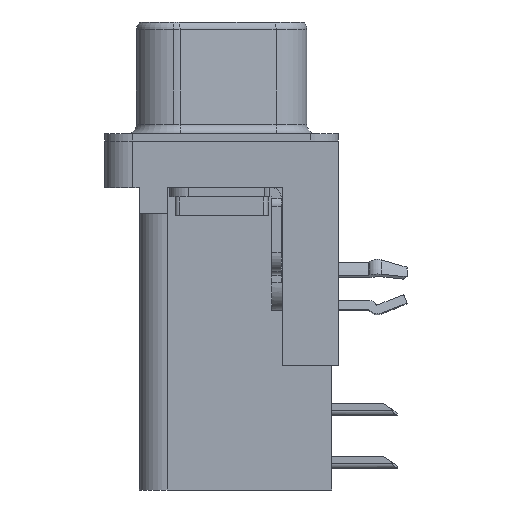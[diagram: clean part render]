
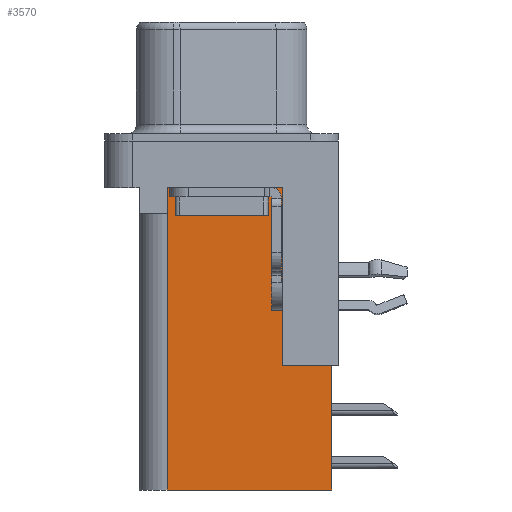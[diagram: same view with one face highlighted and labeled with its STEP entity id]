
A CAD part, left-side view. The second image highlights one B-rep face of the part: STEP entity #3570.
In plain terms, the highlighted planar face has unit normal (-1, 0, 0).
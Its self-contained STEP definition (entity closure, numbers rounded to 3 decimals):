
#552 = VERTEX_POINT ( 'NONE', #10176 ) ;
#607 = VECTOR ( 'NONE', #13355, 1000. ) ;
#747 = LINE ( 'NONE', #12191, #607 ) ;
#1044 = ORIENTED_EDGE ( 'NONE', *, *, #6410, .T. ) ;
#1536 = VECTOR ( 'NONE', #13078, 1000. ) ;
#1740 = LINE ( 'NONE', #16534, #1536 ) ;
#2386 = AXIS2_PLACEMENT_3D ( 'NONE', #10855, #15458, #12419 ) ;
#3159 = ORIENTED_EDGE ( 'NONE', *, *, #15242, .T. ) ;
#3570 = ADVANCED_FACE ( 'NONE', ( #6149 ), #14655, .F. ) ;
#4146 = CARTESIAN_POINT ( 'NONE',  ( 3.765, 2.925, -3.9 ) ) ;
#4366 = DIRECTION ( 'NONE',  ( 0., 0., 1. ) ) ;
#4608 = EDGE_CURVE ( 'NONE', #5738, #17098, #1740, .T. ) ;
#4900 = EDGE_CURVE ( 'NONE', #14322, #7651, #747, .T. ) ;
#4999 = VECTOR ( 'NONE', #13745, 1000. ) ;
#5017 = LINE ( 'NONE', #19969, #4999 ) ;
#5036 = VECTOR ( 'NONE', #10395, 1000. ) ;
#5080 = LINE ( 'NONE', #10647, #5036 ) ;
#5152 = ORIENTED_EDGE ( 'NONE', *, *, #4608, .F. ) ;
#5738 = VERTEX_POINT ( 'NONE', #12251 ) ;
#6149 = FACE_OUTER_BOUND ( 'NONE', #19801, .T. ) ;
#6338 = EDGE_CURVE ( 'NONE', #12247, #6940, #16117, .T. ) ;
#6410 = EDGE_CURVE ( 'NONE', #12247, #552, #15913, .T. ) ;
#6684 = EDGE_CURVE ( 'NONE', #552, #9245, #14926, .T. ) ;
#6762 = ORIENTED_EDGE ( 'NONE', *, *, #11816, .F. ) ;
#6940 = VERTEX_POINT ( 'NONE', #13291 ) ;
#7565 = CARTESIAN_POINT ( 'NONE',  ( 3.765, -3.295, -18.76 ) ) ;
#7651 = VERTEX_POINT ( 'NONE', #13433 ) ;
#7776 = CARTESIAN_POINT ( 'NONE',  ( 3.765, -5.925, -12.05 ) ) ;
#9237 = EDGE_CURVE ( 'NONE', #7651, #17098, #5080, .T. ) ;
#9245 = VERTEX_POINT ( 'NONE', #10326 ) ;
#10036 = CARTESIAN_POINT ( 'NONE',  ( 3.765, -3.295, -18.76 ) ) ;
#10176 = CARTESIAN_POINT ( 'NONE',  ( 3.765, -3.295, -12.05 ) ) ;
#10326 = CARTESIAN_POINT ( 'NONE',  ( 3.765, -3.295, -2.5 ) ) ;
#10370 = ORIENTED_EDGE ( 'NONE', *, *, #6338, .F. ) ;
#10395 = DIRECTION ( 'NONE',  ( 0., 1., 0. ) ) ;
#10647 = CARTESIAN_POINT ( 'NONE',  ( 3.765, 0., -3.9 ) ) ;
#10855 = CARTESIAN_POINT ( 'NONE',  ( 3.765, -3.295, -18.76 ) ) ;
#11762 = DIRECTION ( 'NONE',  ( 0., 1., 0. ) ) ;
#11816 = EDGE_CURVE ( 'NONE', #6940, #5738, #16955, .T. ) ;
#12191 = CARTESIAN_POINT ( 'NONE',  ( 3.765, 2.895, -3.9 ) ) ;
#12247 = VERTEX_POINT ( 'NONE', #7776 ) ;
#12251 = CARTESIAN_POINT ( 'NONE',  ( 3.765, 2.925, -18.76 ) ) ;
#12419 = DIRECTION ( 'NONE',  ( 0., 1., 0. ) ) ;
#13022 = CARTESIAN_POINT ( 'NONE',  ( 3.765, -6.295, -12.05 ) ) ;
#13078 = DIRECTION ( 'NONE',  ( 0., 0., 1. ) ) ;
#13291 = CARTESIAN_POINT ( 'NONE',  ( 3.765, -5.925, -18.76 ) ) ;
#13355 = DIRECTION ( 'NONE',  ( 0., 0., -1. ) ) ;
#13433 = CARTESIAN_POINT ( 'NONE',  ( 3.765, 2.895, -3.9 ) ) ;
#13745 = DIRECTION ( 'NONE',  ( 0., 1., 0. ) ) ;
#14322 = VERTEX_POINT ( 'NONE', #15908 ) ;
#14581 = ORIENTED_EDGE ( 'NONE', *, *, #6684, .T. ) ;
#14655 = PLANE ( 'NONE',  #2386 ) ;
#14926 = LINE ( 'NONE', #7565, #14993 ) ;
#14993 = VECTOR ( 'NONE', #4366, 1000. ) ;
#15242 = EDGE_CURVE ( 'NONE', #9245, #14322, #5017, .T. ) ;
#15458 = DIRECTION ( 'NONE',  ( 1., 0., 0. ) ) ;
#15893 = VECTOR ( 'NONE', #11762, 1000. ) ;
#15908 = CARTESIAN_POINT ( 'NONE',  ( 3.765, 2.895, -2.5 ) ) ;
#15913 = LINE ( 'NONE', #13022, #15893 ) ;
#16068 = VECTOR ( 'NONE', #17858, 1000. ) ;
#16117 = LINE ( 'NONE', #16295, #16068 ) ;
#16295 = CARTESIAN_POINT ( 'NONE',  ( 3.765, -5.925, -2. ) ) ;
#16534 = CARTESIAN_POINT ( 'NONE',  ( 3.765, 2.925, -18.76 ) ) ;
#16935 = VECTOR ( 'NONE', #19464, 1000. ) ;
#16955 = LINE ( 'NONE', #10036, #16935 ) ;
#17098 = VERTEX_POINT ( 'NONE', #4146 ) ;
#17224 = ORIENTED_EDGE ( 'NONE', *, *, #9237, .T. ) ;
#17858 = DIRECTION ( 'NONE',  ( 0., 0., -1. ) ) ;
#19359 = ORIENTED_EDGE ( 'NONE', *, *, #4900, .T. ) ;
#19464 = DIRECTION ( 'NONE',  ( 0., 1., 0. ) ) ;
#19801 = EDGE_LOOP ( 'NONE', ( #3159, #19359, #17224, #5152, #6762, #10370, #1044, #14581 ) ) ;
#19969 = CARTESIAN_POINT ( 'NONE',  ( 3.765, -3.295, -2.5 ) ) ;
